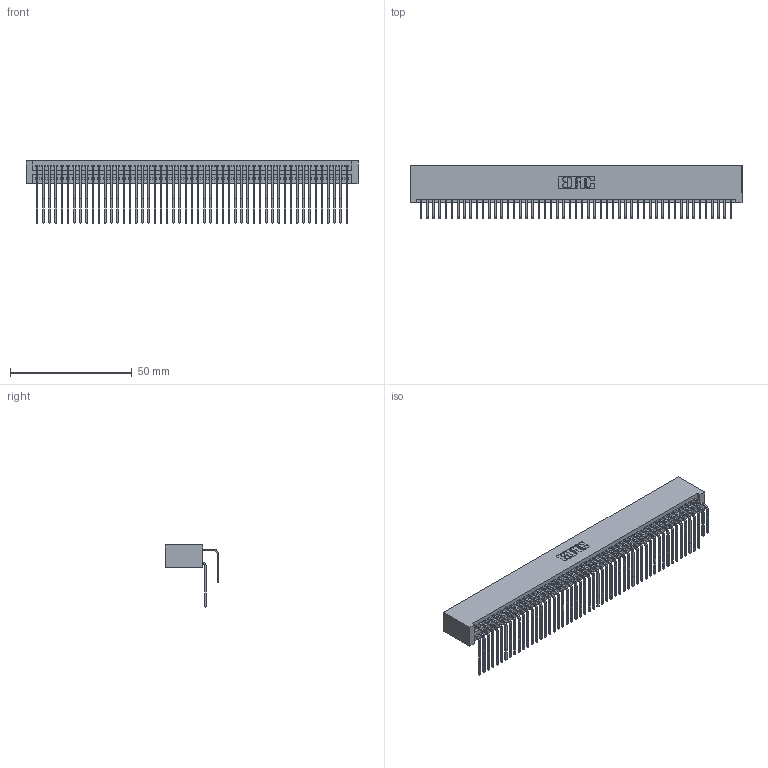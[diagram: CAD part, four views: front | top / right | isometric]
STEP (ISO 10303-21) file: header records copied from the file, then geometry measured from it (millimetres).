
FILE_DESCRIPTION (( 'STEP AP203' ), '1' );
FILE_NAME ('395-102-558-201.STEP', '2019-10-26T19:14:00', ( '' ), ( '' ), 'SwSTEP 2.0', 'SolidWorks 2016', '' );
FILE_SCHEMA (( 'CONFIG_CONTROL_DESIGN' ));
Length unit declared in the file: inch
Products named in the file (4): 345 Part_No Mounting Lugs; 345-292-001_558 559 Tail - 1; 345-292-001_558 Tail - 2; 395-102-558-201
Assembly tree (103 placements, depth 2):
  395-102-558-201
    345 Part_No Mounting Lugs
    345-292-001_558 559 Tail - 1  x51
    345-292-001_558 Tail - 2  x51
Bounding box: 136.14 x 21.83 x 25.53 mm (x, y, z)
Volume: 14513 mm3; surface area: 24697.2 mm2
Topology: 103 solids, 103 shells, 5422 faces, 16127 edges, 10614 vertices
Faces by surface type: plane 3646, cylinder 1776
Entity records: 40179 total; most frequent: CARTESIAN_POINT 6771, ORIENTED_EDGE 6654, DIRECTION 5927, EDGE_CURVE 3327, VECTOR 2959, LINE 2959, VERTEX_POINT 2214, AXIS2_PLACEMENT_3D 1484
